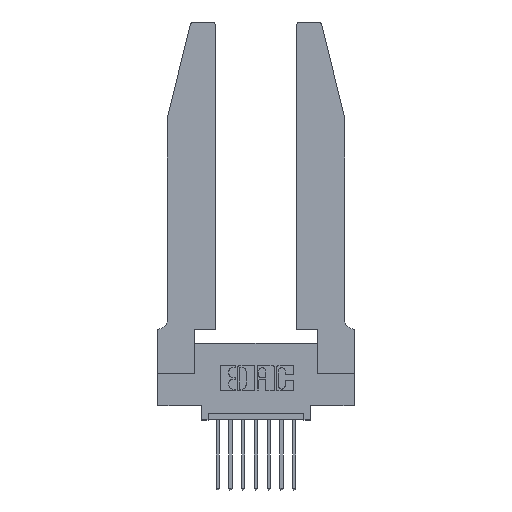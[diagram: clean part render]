
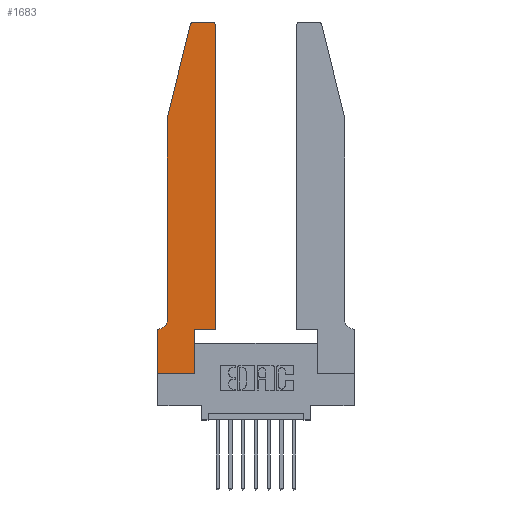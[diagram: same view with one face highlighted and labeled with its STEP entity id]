
A CAD part, top view. The second image highlights one B-rep face of the part: STEP entity #1683.
In plain terms, the highlighted planar face has unit normal (0, 0, 1).
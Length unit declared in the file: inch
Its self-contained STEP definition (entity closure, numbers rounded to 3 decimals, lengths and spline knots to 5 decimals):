
#355 = EDGE_CURVE ( 'NONE', #3713, #6700, #11125, .T. ) ;
#648 = VECTOR ( 'NONE', #8126, 39.37008 ) ;
#769 = ORIENTED_EDGE ( 'NONE', *, *, #2510, .T. ) ;
#781 = VECTOR ( 'NONE', #3630, 39.37008 ) ;
#806 = CARTESIAN_POINT ( 'NONE',  ( 0.2865, 0., 0.37 ) ) ;
#1094 = EDGE_LOOP ( 'NONE', ( #10804, #2884, #769, #14698, #1680, #1273, #1355, #14425, #11470, #10219, #12741, #7933 ) ) ;
#1273 = ORIENTED_EDGE ( 'NONE', *, *, #1559, .T. ) ;
#1355 = ORIENTED_EDGE ( 'NONE', *, *, #13425, .T. ) ;
#1559 = EDGE_CURVE ( 'NONE', #10629, #6565, #11631, .T. ) ;
#1680 = ORIENTED_EDGE ( 'NONE', *, *, #3315, .T. ) ;
#1683 = ADVANCED_FACE ( 'NONE', ( #13830 ), #14645, .T. ) ;
#1792 = CARTESIAN_POINT ( 'NONE',  ( 0.4505, 0.35, 0.37 ) ) ;
#1947 = LINE ( 'NONE', #12379, #13305 ) ;
#2475 = VERTEX_POINT ( 'NONE', #3309 ) ;
#2479 = CARTESIAN_POINT ( 'NONE',  ( 0.284, 2.72, 0.37 ) ) ;
#2510 = EDGE_CURVE ( 'NONE', #12786, #3713, #3716, .T. ) ;
#2656 = VERTEX_POINT ( 'NONE', #12925 ) ;
#2884 = ORIENTED_EDGE ( 'NONE', *, *, #7736, .T. ) ;
#3220 = CARTESIAN_POINT ( 'NONE',  ( 0.4205, 2.75, 0.37 ) ) ;
#3309 = CARTESIAN_POINT ( 'NONE',  ( 0., 0., 0.37 ) ) ;
#3315 = EDGE_CURVE ( 'NONE', #6700, #10629, #11605, .T. ) ;
#3368 = AXIS2_PLACEMENT_3D ( 'NONE', #14609, #5440, #6483 ) ;
#3477 = CARTESIAN_POINT ( 'NONE',  ( 0., 0., 0.37 ) ) ;
#3630 = DIRECTION ( 'NONE',  ( 1., 0., 0. ) ) ;
#3689 = DIRECTION ( 'NONE',  ( -1., 0., 0. ) ) ;
#3713 = VERTEX_POINT ( 'NONE', #7914 ) ;
#3716 = LINE ( 'NONE', #8069, #648 ) ;
#3735 = LINE ( 'NONE', #4459, #11070 ) ;
#4113 = DIRECTION ( 'NONE',  ( 0., 1., 0. ) ) ;
#4120 = DIRECTION ( 'NONE',  ( 1., 0., 0. ) ) ;
#4418 = EDGE_CURVE ( 'NONE', #2475, #11362, #11017, .T. ) ;
#4459 = CARTESIAN_POINT ( 'NONE',  ( 0.2865, 0.35, 0.37 ) ) ;
#4495 = VECTOR ( 'NONE', #3689, 39.37008 ) ;
#4876 = CARTESIAN_POINT ( 'NONE',  ( 0.0055, 0.35, 0.37 ) ) ;
#4974 = VECTOR ( 'NONE', #12708, 39.37008 ) ;
#5308 = CARTESIAN_POINT ( 'NONE',  ( 0.25487, 2.72718, 0.37 ) ) ;
#5440 = DIRECTION ( 'NONE',  ( 0., 0., -1. ) ) ;
#5616 = VERTEX_POINT ( 'NONE', #3220 ) ;
#6483 = DIRECTION ( 'NONE',  ( -1., 0., 0. ) ) ;
#6557 = CARTESIAN_POINT ( 'NONE',  ( 0.0755, 0.42, 0.37 ) ) ;
#6565 = VERTEX_POINT ( 'NONE', #9575 ) ;
#6620 = CIRCLE ( 'NONE', #13247, 0.03 ) ;
#6700 = VERTEX_POINT ( 'NONE', #6557 ) ;
#6764 = CARTESIAN_POINT ( 'NONE',  ( 0.2865, 0.35, 0.37 ) ) ;
#6861 = CARTESIAN_POINT ( 'NONE',  ( 0.4505, 2.72, 0.37 ) ) ;
#6885 = LINE ( 'NONE', #1792, #13939 ) ;
#6952 = DIRECTION ( 'NONE',  ( 0., -1., 0. ) ) ;
#7033 = DIRECTION ( 'NONE',  ( 1., 0., 0. ) ) ;
#7503 = VERTEX_POINT ( 'NONE', #11858 ) ;
#7544 = CARTESIAN_POINT ( 'NONE',  ( 0.0755, 0.35, 0.37 ) ) ;
#7553 = CARTESIAN_POINT ( 'NONE',  ( 0.0755, 2., 0.37 ) ) ;
#7640 = DIRECTION ( 'NONE',  ( 0., 0., 1. ) ) ;
#7683 = DIRECTION ( 'NONE',  ( 1., 0., 0. ) ) ;
#7736 = EDGE_CURVE ( 'NONE', #7503, #12786, #6620, .T. ) ;
#7914 = CARTESIAN_POINT ( 'NONE',  ( 0.0755, 2., 0.37 ) ) ;
#7926 = CARTESIAN_POINT ( 'NONE',  ( 0.4205, 2.72, 0.37 ) ) ;
#7933 = ORIENTED_EDGE ( 'NONE', *, *, #14086, .T. ) ;
#8029 = DIRECTION ( 'NONE',  ( 0., 0., 1. ) ) ;
#8060 = AXIS2_PLACEMENT_3D ( 'NONE', #14601, #7640, #7683 ) ;
#8069 = CARTESIAN_POINT ( 'NONE',  ( 0.0755, 2., 0.37 ) ) ;
#8070 = VECTOR ( 'NONE', #6952, 39.37008 ) ;
#8126 = DIRECTION ( 'NONE',  ( -0.239, -0.971, 0. ) ) ;
#8259 = CARTESIAN_POINT ( 'NONE',  ( 0.4505, 0.35, 0.37 ) ) ;
#8501 = EDGE_CURVE ( 'NONE', #2656, #13527, #11089, .T. ) ;
#8768 = CIRCLE ( 'NONE', #13007, 0.03 ) ;
#8849 = VERTEX_POINT ( 'NONE', #6764 ) ;
#9021 = DIRECTION ( 'NONE',  ( 0., -1., 0. ) ) ;
#9146 = DIRECTION ( 'NONE',  ( 1., 0., 0. ) ) ;
#9575 = CARTESIAN_POINT ( 'NONE',  ( 0., 0.35, 0.37 ) ) ;
#10219 = ORIENTED_EDGE ( 'NONE', *, *, #11320, .T. ) ;
#10629 = VERTEX_POINT ( 'NONE', #4876 ) ;
#10804 = ORIENTED_EDGE ( 'NONE', *, *, #12344, .T. ) ;
#11017 = LINE ( 'NONE', #3477, #781 ) ;
#11070 = VECTOR ( 'NONE', #4113, 39.37008 ) ;
#11089 = LINE ( 'NONE', #8259, #4974 ) ;
#11125 = LINE ( 'NONE', #7553, #8070 ) ;
#11320 = EDGE_CURVE ( 'NONE', #8849, #2656, #6885, .T. ) ;
#11362 = VERTEX_POINT ( 'NONE', #806 ) ;
#11463 = DIRECTION ( 'NONE',  ( 0., 0., 1. ) ) ;
#11470 = ORIENTED_EDGE ( 'NONE', *, *, #14434, .T. ) ;
#11605 = CIRCLE ( 'NONE', #3368, 0.07 ) ;
#11631 = LINE ( 'NONE', #7544, #12530 ) ;
#11858 = CARTESIAN_POINT ( 'NONE',  ( 0.284, 2.75, 0.37 ) ) ;
#12344 = EDGE_CURVE ( 'NONE', #5616, #7503, #12780, .T. ) ;
#12379 = CARTESIAN_POINT ( 'NONE',  ( 0., 0., 0.37 ) ) ;
#12530 = VECTOR ( 'NONE', #14272, 39.37008 ) ;
#12708 = DIRECTION ( 'NONE',  ( 0., 1., 0. ) ) ;
#12741 = ORIENTED_EDGE ( 'NONE', *, *, #8501, .T. ) ;
#12780 = LINE ( 'NONE', #14014, #4495 ) ;
#12786 = VERTEX_POINT ( 'NONE', #5308 ) ;
#12925 = CARTESIAN_POINT ( 'NONE',  ( 0.4505, 0.35, 0.37 ) ) ;
#13007 = AXIS2_PLACEMENT_3D ( 'NONE', #7926, #8029, #7033 ) ;
#13247 = AXIS2_PLACEMENT_3D ( 'NONE', #2479, #11463, #9146 ) ;
#13305 = VECTOR ( 'NONE', #9021, 39.37008 ) ;
#13425 = EDGE_CURVE ( 'NONE', #6565, #2475, #1947, .T. ) ;
#13527 = VERTEX_POINT ( 'NONE', #6861 ) ;
#13830 = FACE_OUTER_BOUND ( 'NONE', #1094, .T. ) ;
#13939 = VECTOR ( 'NONE', #4120, 39.37008 ) ;
#14014 = CARTESIAN_POINT ( 'NONE',  ( 0.2605, 2.75, 0.37 ) ) ;
#14086 = EDGE_CURVE ( 'NONE', #13527, #5616, #8768, .T. ) ;
#14272 = DIRECTION ( 'NONE',  ( -1., 0., 0. ) ) ;
#14425 = ORIENTED_EDGE ( 'NONE', *, *, #4418, .T. ) ;
#14434 = EDGE_CURVE ( 'NONE', #11362, #8849, #3735, .T. ) ;
#14601 = CARTESIAN_POINT ( 'NONE',  ( 0., 0.35, 0.37 ) ) ;
#14609 = CARTESIAN_POINT ( 'NONE',  ( 0.0055, 0.42, 0.37 ) ) ;
#14645 = PLANE ( 'NONE',  #8060 ) ;
#14698 = ORIENTED_EDGE ( 'NONE', *, *, #355, .T. ) ;
